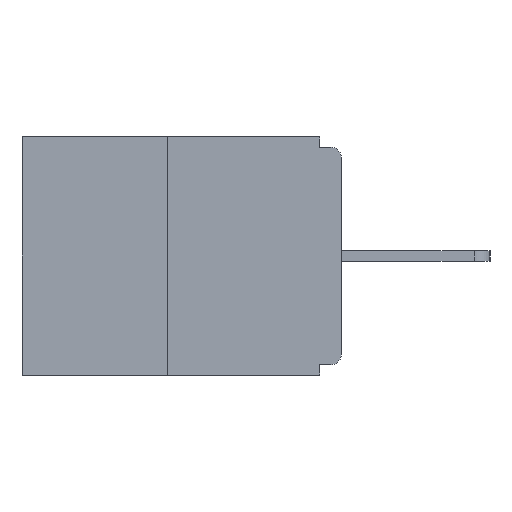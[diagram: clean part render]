
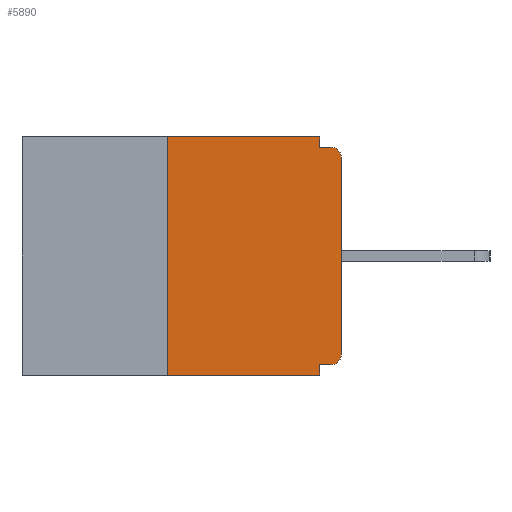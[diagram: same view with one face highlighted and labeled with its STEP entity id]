
A CAD part, left-side view. The second image highlights one B-rep face of the part: STEP entity #5890.
In plain terms, the highlighted planar face has unit normal (-1, 0, 0).
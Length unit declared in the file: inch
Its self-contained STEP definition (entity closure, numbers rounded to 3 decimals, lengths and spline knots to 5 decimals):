
#36 = DIRECTION ( 'NONE',  ( 0., 0., -1. ) ) ;
#201 = CARTESIAN_POINT ( 'NONE',  ( 0., 0.25, 0. ) ) ;
#518 = DIRECTION ( 'NONE',  ( 0., 0., 1. ) ) ;
#785 = CARTESIAN_POINT ( 'NONE',  ( 0., 0.25, 0. ) ) ;
#897 = ORIENTED_EDGE ( 'NONE', *, *, #10710, .T. ) ;
#988 = LINE ( 'NONE', #6515, #12297 ) ;
#1680 = VECTOR ( 'NONE', #14581, 39.37008 ) ;
#1684 = VERTEX_POINT ( 'NONE', #7903 ) ;
#1769 = CARTESIAN_POINT ( 'NONE',  ( 0., 0.031, 0. ) ) ;
#1791 = AXIS2_PLACEMENT_3D ( 'NONE', #2048, #11724, #10372 ) ;
#1905 = CIRCLE ( 'NONE', #15474, 0.015 ) ;
#2048 = CARTESIAN_POINT ( 'NONE',  ( 0., 0.015, -0.313 ) ) ;
#2134 = ORIENTED_EDGE ( 'NONE', *, *, #13440, .F. ) ;
#2206 = CARTESIAN_POINT ( 'NONE',  ( 0., 0., -0.313 ) ) ;
#2368 = DIRECTION ( 'NONE',  ( -1., 0., 0. ) ) ;
#2467 = VECTOR ( 'NONE', #15656, 39.37008 ) ;
#2961 = EDGE_CURVE ( 'NONE', #6490, #12623, #988, .T. ) ;
#3376 = DIRECTION ( 'NONE',  ( 0., 0., -1. ) ) ;
#3562 = LINE ( 'NONE', #9071, #1680 ) ;
#3739 = VERTEX_POINT ( 'NONE', #14781 ) ;
#3989 = DIRECTION ( 'NONE',  ( 0., 1., 0. ) ) ;
#4132 = EDGE_LOOP ( 'NONE', ( #2134, #5863, #6059, #13200, #16469, #897, #15953, #16288, #6667, #9686 ) ) ;
#4781 = VECTOR ( 'NONE', #7808, 39.37008 ) ;
#4853 = VERTEX_POINT ( 'NONE', #1769 ) ;
#5511 = EDGE_CURVE ( 'NONE', #1684, #17424, #3562, .T. ) ;
#5863 = ORIENTED_EDGE ( 'NONE', *, *, #14344, .F. ) ;
#5890 = ADVANCED_FACE ( 'NONE', ( #6259 ), #10583, .F. ) ;
#6059 = ORIENTED_EDGE ( 'NONE', *, *, #5511, .T. ) ;
#6105 = CARTESIAN_POINT ( 'NONE',  ( 0., 0.015, -0.328 ) ) ;
#6141 = VECTOR ( 'NONE', #13882, 39.37008 ) ;
#6182 = LINE ( 'NONE', #15937, #4781 ) ;
#6259 = FACE_OUTER_BOUND ( 'NONE', #4132, .T. ) ;
#6332 = AXIS2_PLACEMENT_3D ( 'NONE', #17101, #15746, #3376 ) ;
#6490 = VERTEX_POINT ( 'NONE', #6105 ) ;
#6515 = CARTESIAN_POINT ( 'NONE',  ( 0., 0., -0.328 ) ) ;
#6667 = ORIENTED_EDGE ( 'NONE', *, *, #13985, .F. ) ;
#6937 = CARTESIAN_POINT ( 'NONE',  ( 0., 0.015, -0.015 ) ) ;
#7221 = LINE ( 'NONE', #12716, #16593 ) ;
#7808 = DIRECTION ( 'NONE',  ( 0., -1., 0. ) ) ;
#7903 = CARTESIAN_POINT ( 'NONE',  ( 0., 0.25, -0.343 ) ) ;
#7954 = VECTOR ( 'NONE', #36, 39.37008 ) ;
#8372 = CARTESIAN_POINT ( 'NONE',  ( 0., 0.031, -0.343 ) ) ;
#8657 = CARTESIAN_POINT ( 'NONE',  ( 0., 0.46, 0. ) ) ;
#8980 = CARTESIAN_POINT ( 'NONE',  ( 0., 0.015, -0.03 ) ) ;
#9071 = CARTESIAN_POINT ( 'NONE',  ( 0., 0.46, -0.343 ) ) ;
#9686 = ORIENTED_EDGE ( 'NONE', *, *, #13830, .F. ) ;
#10372 = DIRECTION ( 'NONE',  ( 0., 0., -1. ) ) ;
#10583 = PLANE ( 'NONE',  #6332 ) ;
#10710 = EDGE_CURVE ( 'NONE', #6490, #17109, #12469, .T. ) ;
#10750 = VERTEX_POINT ( 'NONE', #785 ) ;
#10977 = EDGE_CURVE ( 'NONE', #12623, #17424, #15242, .T. ) ;
#11427 = CARTESIAN_POINT ( 'NONE',  ( 0., 0.031, -0.328 ) ) ;
#11693 = VECTOR ( 'NONE', #14250, 39.37008 ) ;
#11724 = DIRECTION ( 'NONE',  ( -1., 0., 0. ) ) ;
#12297 = VECTOR ( 'NONE', #3989, 39.37008 ) ;
#12469 = CIRCLE ( 'NONE', #1791, 0.015 ) ;
#12578 = LINE ( 'NONE', #201, #2467 ) ;
#12623 = VERTEX_POINT ( 'NONE', #11427 ) ;
#12716 = CARTESIAN_POINT ( 'NONE',  ( 0., 0., 0. ) ) ;
#13200 = ORIENTED_EDGE ( 'NONE', *, *, #10977, .F. ) ;
#13218 = DIRECTION ( 'NONE',  ( 0., 0., -1. ) ) ;
#13440 = EDGE_CURVE ( 'NONE', #10750, #4853, #15427, .T. ) ;
#13511 = EDGE_CURVE ( 'NONE', #17109, #3739, #7221, .T. ) ;
#13694 = CARTESIAN_POINT ( 'NONE',  ( 0., 0.031, 0. ) ) ;
#13783 = CARTESIAN_POINT ( 'NONE',  ( 0., 0.031, -0.343 ) ) ;
#13830 = EDGE_CURVE ( 'NONE', #4853, #17116, #16671, .T. ) ;
#13882 = DIRECTION ( 'NONE',  ( 0., 0., -1. ) ) ;
#13985 = EDGE_CURVE ( 'NONE', #17116, #15738, #6182, .T. ) ;
#14250 = DIRECTION ( 'NONE',  ( 0., -1., 0. ) ) ;
#14335 = CARTESIAN_POINT ( 'NONE',  ( 0., 0.031, -0.015 ) ) ;
#14344 = EDGE_CURVE ( 'NONE', #1684, #10750, #12578, .T. ) ;
#14522 = EDGE_CURVE ( 'NONE', #3739, #15738, #1905, .T. ) ;
#14581 = DIRECTION ( 'NONE',  ( 0., -1., 0. ) ) ;
#14781 = CARTESIAN_POINT ( 'NONE',  ( 0., 0., -0.03 ) ) ;
#15242 = LINE ( 'NONE', #8372, #6141 ) ;
#15427 = LINE ( 'NONE', #8657, #11693 ) ;
#15474 = AXIS2_PLACEMENT_3D ( 'NONE', #8980, #2368, #13218 ) ;
#15656 = DIRECTION ( 'NONE',  ( 0., 0., 1. ) ) ;
#15738 = VERTEX_POINT ( 'NONE', #6937 ) ;
#15746 = DIRECTION ( 'NONE',  ( 1., 0., 0. ) ) ;
#15937 = CARTESIAN_POINT ( 'NONE',  ( 0., 0., -0.015 ) ) ;
#15953 = ORIENTED_EDGE ( 'NONE', *, *, #13511, .T. ) ;
#16288 = ORIENTED_EDGE ( 'NONE', *, *, #14522, .T. ) ;
#16469 = ORIENTED_EDGE ( 'NONE', *, *, #2961, .F. ) ;
#16593 = VECTOR ( 'NONE', #518, 39.37008 ) ;
#16671 = LINE ( 'NONE', #13694, #7954 ) ;
#17101 = CARTESIAN_POINT ( 'NONE',  ( 0., 0.46, 0. ) ) ;
#17109 = VERTEX_POINT ( 'NONE', #2206 ) ;
#17116 = VERTEX_POINT ( 'NONE', #14335 ) ;
#17424 = VERTEX_POINT ( 'NONE', #13783 ) ;
